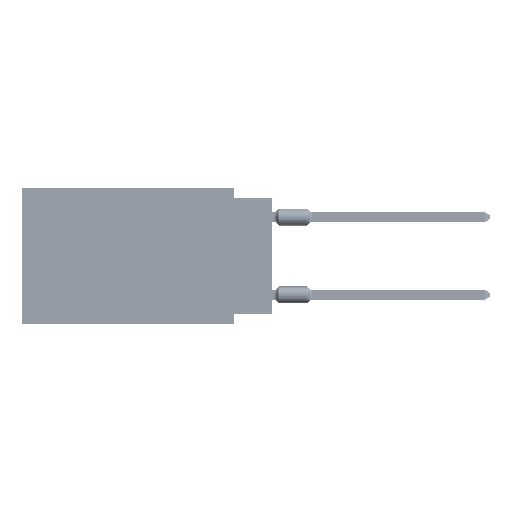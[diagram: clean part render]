
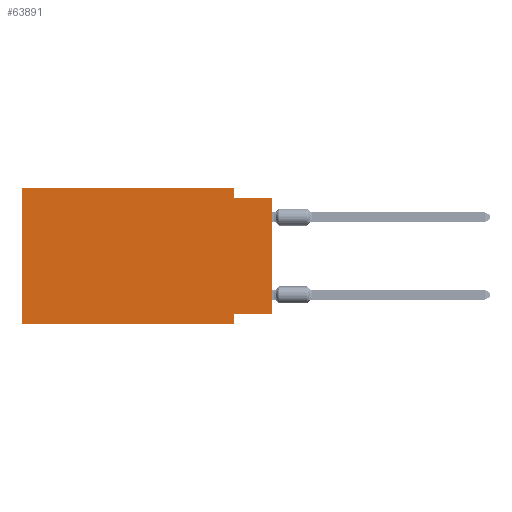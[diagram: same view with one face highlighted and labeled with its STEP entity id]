
A CAD part, left-side view. The second image highlights one B-rep face of the part: STEP entity #63891.
In plain terms, the highlighted planar face has unit normal (-1, 0, 0).
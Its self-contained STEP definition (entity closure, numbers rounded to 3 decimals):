
#612 = DIRECTION ( 'NONE',  ( 0., 0., 1. ) ) ;
#1098 = VERTEX_POINT ( 'NONE', #43700 ) ;
#1101 = LINE ( 'NONE', #51185, #55367 ) ;
#1966 = DIRECTION ( 'NONE',  ( 0., 0., -1. ) ) ;
#2975 = CARTESIAN_POINT ( 'NONE',  ( 0., 0., -0.635 ) ) ;
#4394 = VECTOR ( 'NONE', #1966, 1000. ) ;
#4524 = DIRECTION ( 'NONE',  ( 0., 0., -1. ) ) ;
#5648 = EDGE_CURVE ( 'NONE', #31139, #53822, #33585, .T. ) ;
#6089 = CARTESIAN_POINT ( 'NONE',  ( 0., 16.383, 0. ) ) ;
#6811 = CARTESIAN_POINT ( 'NONE',  ( 0., 16.383, 0. ) ) ;
#7441 = CARTESIAN_POINT ( 'NONE',  ( 0., 2.54, -0.635 ) ) ;
#8101 = LINE ( 'NONE', #64387, #59605 ) ;
#8169 = CARTESIAN_POINT ( 'NONE',  ( 0., 2.54, -8.89 ) ) ;
#8211 = ORIENTED_EDGE ( 'NONE', *, *, #5648, .T. ) ;
#8453 = DIRECTION ( 'NONE',  ( 0., 0., -1. ) ) ;
#10493 = VECTOR ( 'NONE', #612, 1000. ) ;
#12424 = CARTESIAN_POINT ( 'NONE',  ( 0., 0., -0.635 ) ) ;
#13956 = LINE ( 'NONE', #2975, #16016 ) ;
#14001 = EDGE_CURVE ( 'NONE', #36878, #29262, #1101, .T. ) ;
#15428 = VECTOR ( 'NONE', #69008, 1000. ) ;
#16016 = VECTOR ( 'NONE', #64397, 1000. ) ;
#17408 = EDGE_CURVE ( 'NONE', #36878, #32668, #57673, .T. ) ;
#17758 = LINE ( 'NONE', #6811, #10493 ) ;
#21424 = CARTESIAN_POINT ( 'NONE',  ( 0., 16.383, -8.89 ) ) ;
#22575 = EDGE_CURVE ( 'NONE', #32668, #53822, #64821, .T. ) ;
#24398 = CARTESIAN_POINT ( 'NONE',  ( 0., 0., -8.255 ) ) ;
#25727 = FACE_OUTER_BOUND ( 'NONE', #60841, .T. ) ;
#29171 = CARTESIAN_POINT ( 'NONE',  ( 0., 16.383, 0. ) ) ;
#29262 = VERTEX_POINT ( 'NONE', #12424 ) ;
#30888 = ORIENTED_EDGE ( 'NONE', *, *, #17408, .F. ) ;
#31139 = VERTEX_POINT ( 'NONE', #21424 ) ;
#32668 = VERTEX_POINT ( 'NONE', #47723 ) ;
#33015 = PLANE ( 'NONE',  #58795 ) ;
#33585 = LINE ( 'NONE', #66502, #40002 ) ;
#33691 = ORIENTED_EDGE ( 'NONE', *, *, #34714, .F. ) ;
#33741 = VERTEX_POINT ( 'NONE', #6089 ) ;
#34714 = EDGE_CURVE ( 'NONE', #1098, #60013, #8101, .T. ) ;
#35002 = ORIENTED_EDGE ( 'NONE', *, *, #14001, .T. ) ;
#36878 = VERTEX_POINT ( 'NONE', #52465 ) ;
#38517 = CARTESIAN_POINT ( 'NONE',  ( 0., 16.383, 0. ) ) ;
#38859 = ORIENTED_EDGE ( 'NONE', *, *, #54198, .F. ) ;
#40002 = VECTOR ( 'NONE', #66141, 1000. ) ;
#41661 = VECTOR ( 'NONE', #51474, 1000. ) ;
#43700 = CARTESIAN_POINT ( 'NONE',  ( 0., 2.54, 0. ) ) ;
#44372 = ORIENTED_EDGE ( 'NONE', *, *, #50158, .F. ) ;
#47723 = CARTESIAN_POINT ( 'NONE',  ( 0., 2.54, -8.255 ) ) ;
#50158 = EDGE_CURVE ( 'NONE', #60013, #29262, #13956, .T. ) ;
#51185 = CARTESIAN_POINT ( 'NONE',  ( 0., 0., 0. ) ) ;
#51474 = DIRECTION ( 'NONE',  ( 0., -1., 0. ) ) ;
#52465 = CARTESIAN_POINT ( 'NONE',  ( 0., 0., -8.255 ) ) ;
#53571 = ORIENTED_EDGE ( 'NONE', *, *, #22575, .F. ) ;
#53822 = VERTEX_POINT ( 'NONE', #64334 ) ;
#54198 = EDGE_CURVE ( 'NONE', #33741, #1098, #62459, .T. ) ;
#54617 = DIRECTION ( 'NONE',  ( 1., 0., 0. ) ) ;
#55367 = VECTOR ( 'NONE', #55945, 1000. ) ;
#55945 = DIRECTION ( 'NONE',  ( 0., 0., 1. ) ) ;
#57673 = LINE ( 'NONE', #24398, #15428 ) ;
#58795 = AXIS2_PLACEMENT_3D ( 'NONE', #38517, #54617, #4524 ) ;
#59405 = EDGE_CURVE ( 'NONE', #31139, #33741, #17758, .T. ) ;
#59605 = VECTOR ( 'NONE', #8453, 1000. ) ;
#60013 = VERTEX_POINT ( 'NONE', #7441 ) ;
#60727 = ORIENTED_EDGE ( 'NONE', *, *, #59405, .F. ) ;
#60841 = EDGE_LOOP ( 'NONE', ( #35002, #44372, #33691, #38859, #60727, #8211, #53571, #30888 ) ) ;
#62459 = LINE ( 'NONE', #29171, #41661 ) ;
#63891 = ADVANCED_FACE ( 'NONE', ( #25727 ), #33015, .F. ) ;
#64334 = CARTESIAN_POINT ( 'NONE',  ( 0., 2.54, -8.89 ) ) ;
#64387 = CARTESIAN_POINT ( 'NONE',  ( 0., 2.54, 0. ) ) ;
#64397 = DIRECTION ( 'NONE',  ( 0., -1., 0. ) ) ;
#64821 = LINE ( 'NONE', #8169, #4394 ) ;
#66141 = DIRECTION ( 'NONE',  ( 0., -1., 0. ) ) ;
#66502 = CARTESIAN_POINT ( 'NONE',  ( 0., 16.383, -8.89 ) ) ;
#69008 = DIRECTION ( 'NONE',  ( 0., 1., 0. ) ) ;
